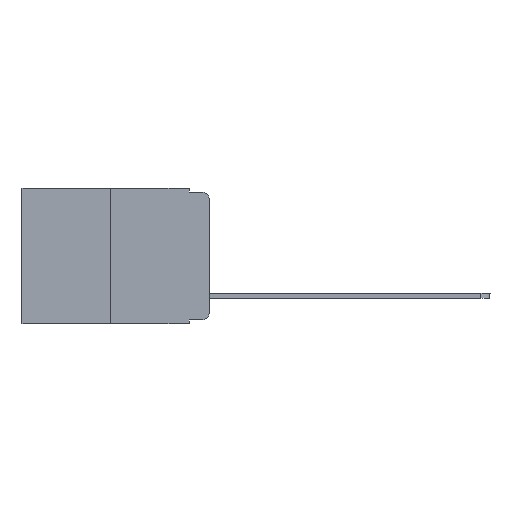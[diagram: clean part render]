
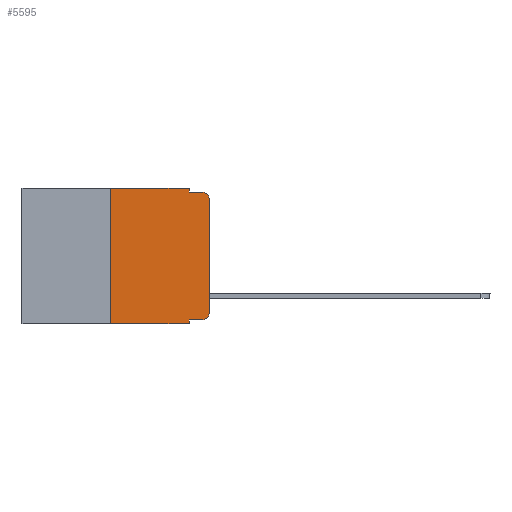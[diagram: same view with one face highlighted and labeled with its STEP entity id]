
A CAD part, left-side view. The second image highlights one B-rep face of the part: STEP entity #5595.
In plain terms, the highlighted planar face has unit normal (-1, 0, 0).
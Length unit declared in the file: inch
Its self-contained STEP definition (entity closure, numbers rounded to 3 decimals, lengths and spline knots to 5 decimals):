
#405 = VECTOR ( 'NONE', #3527, 39.37008 ) ;
#575 = CARTESIAN_POINT ( 'NONE',  ( 0., 0.25, -0.343 ) ) ;
#601 = CARTESIAN_POINT ( 'NONE',  ( 0., 0.051, 0. ) ) ;
#1034 = LINE ( 'NONE', #5063, #10983 ) ;
#1066 = CARTESIAN_POINT ( 'NONE',  ( 0., 0., -0.03 ) ) ;
#1074 = DIRECTION ( 'NONE',  ( 0., 0., -1. ) ) ;
#1093 = CARTESIAN_POINT ( 'NONE',  ( 0., 0., 0. ) ) ;
#1436 = DIRECTION ( 'NONE',  ( -1., 0., 0. ) ) ;
#1440 = EDGE_CURVE ( 'NONE', #9699, #6581, #5958, .T. ) ;
#1727 = CIRCLE ( 'NONE', #2969, 0.02 ) ;
#1821 = ORIENTED_EDGE ( 'NONE', *, *, #1440, .T. ) ;
#1837 = DIRECTION ( 'NONE',  ( 0., 0., -1. ) ) ;
#2246 = CARTESIAN_POINT ( 'NONE',  ( 0., 0.051, -0.333 ) ) ;
#2786 = CARTESIAN_POINT ( 'NONE',  ( 0., 0.25, 0. ) ) ;
#2790 = AXIS2_PLACEMENT_3D ( 'NONE', #13551, #9389, #1074 ) ;
#2969 = AXIS2_PLACEMENT_3D ( 'NONE', #9756, #1436, #11164 ) ;
#2999 = CARTESIAN_POINT ( 'NONE',  ( 0., 0., -0.313 ) ) ;
#3353 = ORIENTED_EDGE ( 'NONE', *, *, #12094, .T. ) ;
#3463 = CARTESIAN_POINT ( 'NONE',  ( 0., 0.473, 0. ) ) ;
#3527 = DIRECTION ( 'NONE',  ( 0., -1., 0. ) ) ;
#3802 = CARTESIAN_POINT ( 'NONE',  ( 0., 0.473, -0.343 ) ) ;
#3862 = VERTEX_POINT ( 'NONE', #1066 ) ;
#3925 = DIRECTION ( 'NONE',  ( 1., 0., 0. ) ) ;
#4031 = VERTEX_POINT ( 'NONE', #7266 ) ;
#4080 = EDGE_CURVE ( 'NONE', #16721, #15454, #7701, .T. ) ;
#4107 = LINE ( 'NONE', #2246, #405 ) ;
#4128 = VERTEX_POINT ( 'NONE', #4338 ) ;
#4262 = VERTEX_POINT ( 'NONE', #575 ) ;
#4338 = CARTESIAN_POINT ( 'NONE',  ( 0., 0.051, 0. ) ) ;
#4752 = ORIENTED_EDGE ( 'NONE', *, *, #12583, .T. ) ;
#4812 = VECTOR ( 'NONE', #1837, 39.37008 ) ;
#5063 = CARTESIAN_POINT ( 'NONE',  ( 0., 0.051, 0. ) ) ;
#5426 = DIRECTION ( 'NONE',  ( 0., 0., -1. ) ) ;
#5518 = ORIENTED_EDGE ( 'NONE', *, *, #4080, .F. ) ;
#5595 = ADVANCED_FACE ( 'NONE', ( #7440 ), #17652, .F. ) ;
#5958 = CIRCLE ( 'NONE', #2790, 0.02 ) ;
#6370 = CARTESIAN_POINT ( 'NONE',  ( 0., 0.051, -0.343 ) ) ;
#6404 = VECTOR ( 'NONE', #9880, 39.37008 ) ;
#6419 = LINE ( 'NONE', #3463, #7725 ) ;
#6544 = VECTOR ( 'NONE', #6966, 39.37008 ) ;
#6581 = VERTEX_POINT ( 'NONE', #2999 ) ;
#6653 = CARTESIAN_POINT ( 'NONE',  ( 0., 0.473, 0. ) ) ;
#6726 = CARTESIAN_POINT ( 'NONE',  ( 0., 0.051, -0.01 ) ) ;
#6826 = ORIENTED_EDGE ( 'NONE', *, *, #10675, .F. ) ;
#6966 = DIRECTION ( 'NONE',  ( 0., 0., 1. ) ) ;
#7266 = CARTESIAN_POINT ( 'NONE',  ( 0., 0.25, 0. ) ) ;
#7418 = DIRECTION ( 'NONE',  ( 0., -1., 0. ) ) ;
#7440 = FACE_OUTER_BOUND ( 'NONE', #13399, .T. ) ;
#7491 = EDGE_CURVE ( 'NONE', #3862, #15454, #1727, .T. ) ;
#7628 = LINE ( 'NONE', #3802, #15511 ) ;
#7701 = LINE ( 'NONE', #8404, #6404 ) ;
#7725 = VECTOR ( 'NONE', #7418, 39.37008 ) ;
#7824 = ORIENTED_EDGE ( 'NONE', *, *, #11013, .F. ) ;
#8249 = EDGE_CURVE ( 'NONE', #4031, #4128, #6419, .T. ) ;
#8404 = CARTESIAN_POINT ( 'NONE',  ( 0., 0.051, -0.01 ) ) ;
#8406 = VERTEX_POINT ( 'NONE', #6370 ) ;
#8537 = ORIENTED_EDGE ( 'NONE', *, *, #14365, .F. ) ;
#8867 = CARTESIAN_POINT ( 'NONE',  ( 0., 0.051, -0.333 ) ) ;
#9389 = DIRECTION ( 'NONE',  ( -1., 0., 0. ) ) ;
#9456 = VERTEX_POINT ( 'NONE', #8867 ) ;
#9699 = VERTEX_POINT ( 'NONE', #12243 ) ;
#9756 = CARTESIAN_POINT ( 'NONE',  ( 0., 0.02, -0.03 ) ) ;
#9880 = DIRECTION ( 'NONE',  ( 0., -1., 0. ) ) ;
#10675 = EDGE_CURVE ( 'NONE', #4128, #16721, #17078, .T. ) ;
#10856 = DIRECTION ( 'NONE',  ( 0., -1., 0. ) ) ;
#10983 = VECTOR ( 'NONE', #17691, 39.37008 ) ;
#11013 = EDGE_CURVE ( 'NONE', #4262, #4031, #17488, .T. ) ;
#11164 = DIRECTION ( 'NONE',  ( 0., 0., -1. ) ) ;
#11195 = ORIENTED_EDGE ( 'NONE', *, *, #11361, .T. ) ;
#11361 = EDGE_CURVE ( 'NONE', #4262, #8406, #7628, .T. ) ;
#11986 = LINE ( 'NONE', #1093, #13918 ) ;
#12094 = EDGE_CURVE ( 'NONE', #6581, #3862, #11986, .T. ) ;
#12243 = CARTESIAN_POINT ( 'NONE',  ( 0., 0.02, -0.333 ) ) ;
#12583 = EDGE_CURVE ( 'NONE', #9456, #9699, #4107, .T. ) ;
#12855 = CARTESIAN_POINT ( 'NONE',  ( 0., 0.02, -0.01 ) ) ;
#13399 = EDGE_LOOP ( 'NONE', ( #3353, #17570, #5518, #6826, #16971, #7824, #11195, #8537, #4752, #1821 ) ) ;
#13551 = CARTESIAN_POINT ( 'NONE',  ( 0., 0.02, -0.313 ) ) ;
#13814 = DIRECTION ( 'NONE',  ( 0., 0., 1. ) ) ;
#13918 = VECTOR ( 'NONE', #13814, 39.37008 ) ;
#14365 = EDGE_CURVE ( 'NONE', #9456, #8406, #1034, .T. ) ;
#15340 = AXIS2_PLACEMENT_3D ( 'NONE', #6653, #3925, #5426 ) ;
#15454 = VERTEX_POINT ( 'NONE', #12855 ) ;
#15511 = VECTOR ( 'NONE', #10856, 39.37008 ) ;
#16721 = VERTEX_POINT ( 'NONE', #6726 ) ;
#16971 = ORIENTED_EDGE ( 'NONE', *, *, #8249, .F. ) ;
#17078 = LINE ( 'NONE', #601, #4812 ) ;
#17488 = LINE ( 'NONE', #2786, #6544 ) ;
#17570 = ORIENTED_EDGE ( 'NONE', *, *, #7491, .T. ) ;
#17652 = PLANE ( 'NONE',  #15340 ) ;
#17691 = DIRECTION ( 'NONE',  ( 0., 0., -1. ) ) ;
